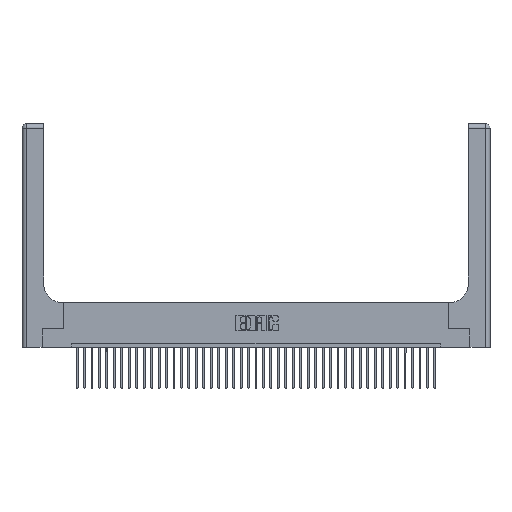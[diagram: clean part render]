
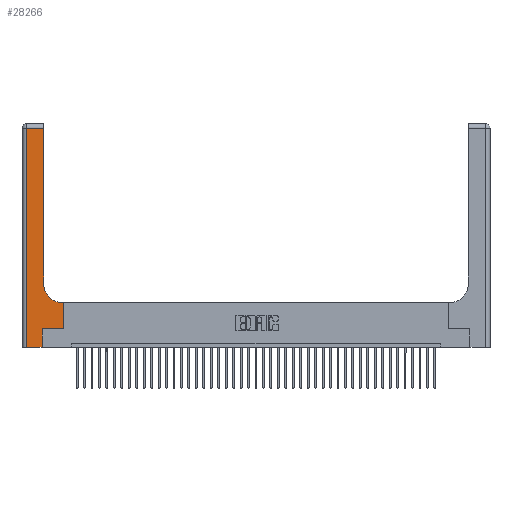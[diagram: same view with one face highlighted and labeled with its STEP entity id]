
A CAD part, top view. The second image highlights one B-rep face of the part: STEP entity #28266.
In plain terms, the highlighted planar face has unit normal (0, 0, 1).
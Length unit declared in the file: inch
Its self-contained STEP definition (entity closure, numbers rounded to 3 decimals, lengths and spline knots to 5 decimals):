
#245 = CARTESIAN_POINT ( 'NONE',  ( 0.5585, 0.25, 0.37 ) ) ;
#580 = DIRECTION ( 'NONE',  ( 0., 0., -1. ) ) ;
#1697 = CARTESIAN_POINT ( 'NONE',  ( 0.2915, 0.6, 0.37 ) ) ;
#2312 = VECTOR ( 'NONE', #3863, 39.37008 ) ;
#2659 = DIRECTION ( 'NONE',  ( 0., 0., -1. ) ) ;
#3863 = DIRECTION ( 'NONE',  ( 0., 1., 0. ) ) ;
#5043 = VECTOR ( 'NONE', #35748, 39.37008 ) ;
#5868 = DIRECTION ( 'NONE',  ( -1., 0., 0. ) ) ;
#6372 = VECTOR ( 'NONE', #23879, 39.37008 ) ;
#7231 = ORIENTED_EDGE ( 'NONE', *, *, #40777, .T. ) ;
#7431 = CARTESIAN_POINT ( 'NONE',  ( 0.2915, 2.94, 0.37 ) ) ;
#7917 = EDGE_CURVE ( 'NONE', #13320, #29492, #40012, .T. ) ;
#8288 = VECTOR ( 'NONE', #13413, 39.37008 ) ;
#8339 = VECTOR ( 'NONE', #39174, 39.37008 ) ;
#8424 = EDGE_CURVE ( 'NONE', #29492, #14238, #21089, .T. ) ;
#8854 = VERTEX_POINT ( 'NONE', #12000 ) ;
#9354 = VECTOR ( 'NONE', #18501, 39.37008 ) ;
#11156 = ORIENTED_EDGE ( 'NONE', *, *, #26491, .T. ) ;
#11991 = PLANE ( 'NONE',  #30967 ) ;
#12000 = CARTESIAN_POINT ( 'NONE',  ( 0.5585, 0.6, 0.37 ) ) ;
#12123 = CARTESIAN_POINT ( 'NONE',  ( 0., 3., 0.37 ) ) ;
#12796 = DIRECTION ( 'NONE',  ( 0., -1., 0. ) ) ;
#13302 = DIRECTION ( 'NONE',  ( 1., 0., 0. ) ) ;
#13320 = VERTEX_POINT ( 'NONE', #32328 ) ;
#13413 = DIRECTION ( 'NONE',  ( 0., 1., 0. ) ) ;
#13861 = CARTESIAN_POINT ( 'NONE',  ( 0.2915, 0.85, 0.37 ) ) ;
#14236 = LINE ( 'NONE', #1697, #6372 ) ;
#14238 = VERTEX_POINT ( 'NONE', #39685 ) ;
#14577 = VERTEX_POINT ( 'NONE', #7431 ) ;
#15385 = FACE_OUTER_BOUND ( 'NONE', #25070, .T. ) ;
#15714 = CARTESIAN_POINT ( 'NONE',  ( 0., 0., 0.37 ) ) ;
#15884 = AXIS2_PLACEMENT_3D ( 'NONE', #26286, #580, #13302 ) ;
#16483 = EDGE_CURVE ( 'NONE', #27273, #8854, #25549, .T. ) ;
#17090 = EDGE_CURVE ( 'NONE', #35435, #35478, #28953, .T. ) ;
#17794 = CARTESIAN_POINT ( 'NONE',  ( 0.06, 2.94, 0.37 ) ) ;
#18170 = LINE ( 'NONE', #34964, #8339 ) ;
#18501 = DIRECTION ( 'NONE',  ( 1., 0., 0. ) ) ;
#18538 = ORIENTED_EDGE ( 'NONE', *, *, #7917, .T. ) ;
#19896 = VECTOR ( 'NONE', #12796, 39.37008 ) ;
#20661 = ORIENTED_EDGE ( 'NONE', *, *, #8424, .T. ) ;
#21089 = LINE ( 'NONE', #37455, #32469 ) ;
#23879 = DIRECTION ( 'NONE',  ( -1., 0., 0. ) ) ;
#24573 = CARTESIAN_POINT ( 'NONE',  ( 0.269, 0., 0.37 ) ) ;
#25070 = EDGE_LOOP ( 'NONE', ( #7231, #25209, #11156, #18538, #20661, #32894, #27590, #29855, #29485 ) ) ;
#25209 = ORIENTED_EDGE ( 'NONE', *, *, #26805, .T. ) ;
#25549 = LINE ( 'NONE', #39672, #8288 ) ;
#26286 = CARTESIAN_POINT ( 'NONE',  ( 0.5415, 0.85, 0.37 ) ) ;
#26491 = EDGE_CURVE ( 'NONE', #31824, #13320, #35751, .T. ) ;
#26805 = EDGE_CURVE ( 'NONE', #14577, #31824, #36793, .T. ) ;
#27273 = VERTEX_POINT ( 'NONE', #245 ) ;
#27590 = ORIENTED_EDGE ( 'NONE', *, *, #16483, .T. ) ;
#28266 = ADVANCED_FACE ( 'NONE', ( #15385 ), #11991, .F. ) ;
#28953 = CIRCLE ( 'NONE', #15884, 0.25 ) ;
#29485 = ORIENTED_EDGE ( 'NONE', *, *, #17090, .T. ) ;
#29492 = VERTEX_POINT ( 'NONE', #24573 ) ;
#29507 = CARTESIAN_POINT ( 'NONE',  ( 0.2915, 3., 0.37 ) ) ;
#29855 = ORIENTED_EDGE ( 'NONE', *, *, #40389, .T. ) ;
#30219 = EDGE_CURVE ( 'NONE', #14238, #27273, #18170, .T. ) ;
#30967 = AXIS2_PLACEMENT_3D ( 'NONE', #12123, #2659, #5868 ) ;
#30972 = DIRECTION ( 'NONE',  ( 0., 1., 0. ) ) ;
#31824 = VERTEX_POINT ( 'NONE', #17794 ) ;
#32328 = CARTESIAN_POINT ( 'NONE',  ( 0.06, 0., 0.37 ) ) ;
#32469 = VECTOR ( 'NONE', #30972, 39.37008 ) ;
#32573 = CARTESIAN_POINT ( 'NONE',  ( 0., 2.94, 0.37 ) ) ;
#32894 = ORIENTED_EDGE ( 'NONE', *, *, #30219, .T. ) ;
#34964 = CARTESIAN_POINT ( 'NONE',  ( 0.269, 0.25, 0.37 ) ) ;
#35435 = VERTEX_POINT ( 'NONE', #36279 ) ;
#35478 = VERTEX_POINT ( 'NONE', #13861 ) ;
#35748 = DIRECTION ( 'NONE',  ( -1., 0., 0. ) ) ;
#35751 = LINE ( 'NONE', #37493, #19896 ) ;
#36279 = CARTESIAN_POINT ( 'NONE',  ( 0.5415, 0.6, 0.37 ) ) ;
#36793 = LINE ( 'NONE', #32573, #5043 ) ;
#37455 = CARTESIAN_POINT ( 'NONE',  ( 0.269, 0., 0.37 ) ) ;
#37493 = CARTESIAN_POINT ( 'NONE',  ( 0.06, 3., 0.37 ) ) ;
#39009 = LINE ( 'NONE', #29507, #2312 ) ;
#39174 = DIRECTION ( 'NONE',  ( 1., 0., 0. ) ) ;
#39672 = CARTESIAN_POINT ( 'NONE',  ( 0.5585, 0.25, 0.37 ) ) ;
#39685 = CARTESIAN_POINT ( 'NONE',  ( 0.269, 0.25, 0.37 ) ) ;
#40012 = LINE ( 'NONE', #15714, #9354 ) ;
#40389 = EDGE_CURVE ( 'NONE', #8854, #35435, #14236, .T. ) ;
#40777 = EDGE_CURVE ( 'NONE', #35478, #14577, #39009, .T. ) ;
